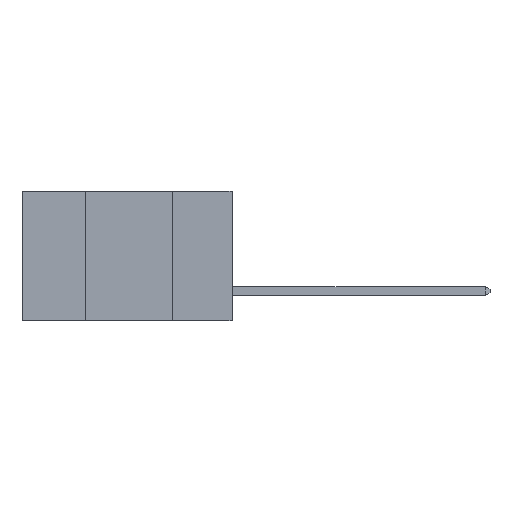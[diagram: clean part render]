
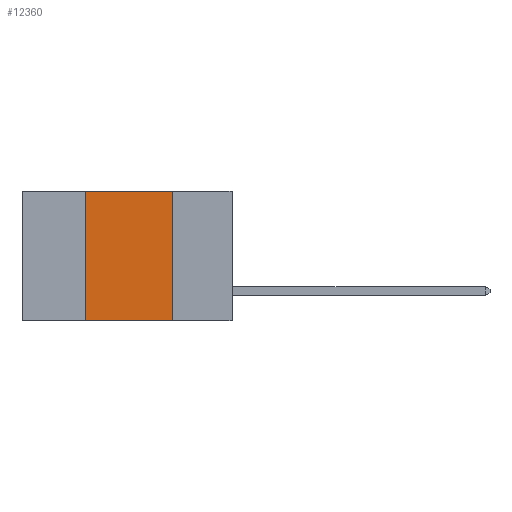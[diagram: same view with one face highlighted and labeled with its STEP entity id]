
A CAD part, left-side view. The second image highlights one B-rep face of the part: STEP entity #12360.
In plain terms, the highlighted planar face has unit normal (-1, 0, 0).
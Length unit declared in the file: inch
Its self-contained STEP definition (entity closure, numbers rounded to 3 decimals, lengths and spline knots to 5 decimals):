
#803 = CARTESIAN_POINT ( 'NONE',  ( 0., 0.6, 0. ) ) ;
#1054 = VECTOR ( 'NONE', #8418, 39.37008 ) ;
#1156 = EDGE_CURVE ( 'NONE', #12217, #5881, #8566, .T. ) ;
#1616 = VERTEX_POINT ( 'NONE', #15377 ) ;
#2362 = LINE ( 'NONE', #22364, #12162 ) ;
#2608 = VECTOR ( 'NONE', #8294, 39.37008 ) ;
#3198 = EDGE_LOOP ( 'NONE', ( #20028, #21287, #8498, #18783 ) ) ;
#3715 = PLANE ( 'NONE',  #14385 ) ;
#5352 = CARTESIAN_POINT ( 'NONE',  ( 0., 0.42, -0.37 ) ) ;
#5546 = LINE ( 'NONE', #803, #14597 ) ;
#5881 = VERTEX_POINT ( 'NONE', #10776 ) ;
#6470 = CARTESIAN_POINT ( 'NONE',  ( 0., 0.42, 0. ) ) ;
#8294 = DIRECTION ( 'NONE',  ( 0., 0., -1. ) ) ;
#8418 = DIRECTION ( 'NONE',  ( 0., 0., 1. ) ) ;
#8498 = ORIENTED_EDGE ( 'NONE', *, *, #25254, .F. ) ;
#8566 = LINE ( 'NONE', #12009, #2608 ) ;
#9690 = DIRECTION ( 'NONE',  ( 1., 0., 0. ) ) ;
#10776 = CARTESIAN_POINT ( 'NONE',  ( 0., 0.17, -0.37 ) ) ;
#11535 = EDGE_CURVE ( 'NONE', #1616, #12217, #5546, .T. ) ;
#12009 = CARTESIAN_POINT ( 'NONE',  ( 0., 0.17, 0. ) ) ;
#12162 = VECTOR ( 'NONE', #24325, 39.37008 ) ;
#12217 = VERTEX_POINT ( 'NONE', #14941 ) ;
#12360 = ADVANCED_FACE ( 'NONE', ( #20399 ), #3715, .F. ) ;
#12514 = DIRECTION ( 'NONE',  ( 0., -1., 0. ) ) ;
#14385 = AXIS2_PLACEMENT_3D ( 'NONE', #21321, #9690, #23297 ) ;
#14597 = VECTOR ( 'NONE', #12514, 39.37008 ) ;
#14941 = CARTESIAN_POINT ( 'NONE',  ( 0., 0.17, 0. ) ) ;
#15377 = CARTESIAN_POINT ( 'NONE',  ( 0., 0.42, 0. ) ) ;
#17246 = VERTEX_POINT ( 'NONE', #5352 ) ;
#18783 = ORIENTED_EDGE ( 'NONE', *, *, #23967, .T. ) ;
#20028 = ORIENTED_EDGE ( 'NONE', *, *, #1156, .F. ) ;
#20399 = FACE_OUTER_BOUND ( 'NONE', #3198, .T. ) ;
#21287 = ORIENTED_EDGE ( 'NONE', *, *, #11535, .F. ) ;
#21321 = CARTESIAN_POINT ( 'NONE',  ( 0., 0.6, 0. ) ) ;
#21904 = LINE ( 'NONE', #6470, #1054 ) ;
#22364 = CARTESIAN_POINT ( 'NONE',  ( 0., 0.6, -0.37 ) ) ;
#23297 = DIRECTION ( 'NONE',  ( 0., 0., -1. ) ) ;
#23967 = EDGE_CURVE ( 'NONE', #17246, #5881, #2362, .T. ) ;
#24325 = DIRECTION ( 'NONE',  ( 0., -1., 0. ) ) ;
#25254 = EDGE_CURVE ( 'NONE', #17246, #1616, #21904, .T. ) ;
